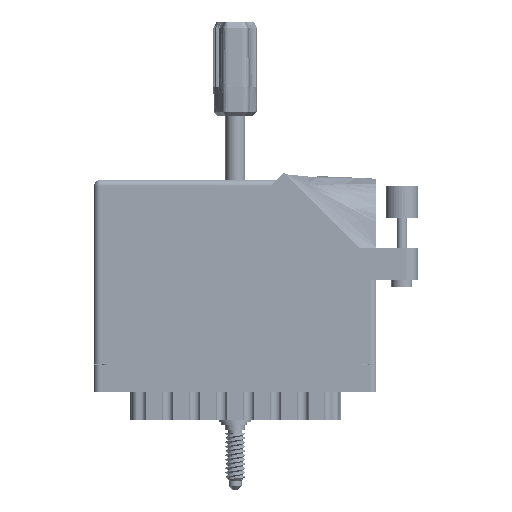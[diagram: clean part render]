
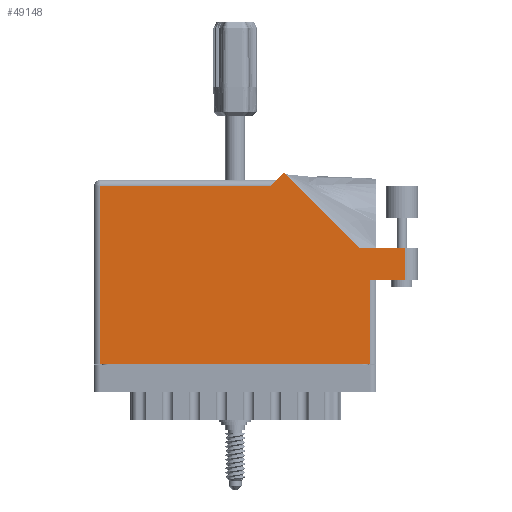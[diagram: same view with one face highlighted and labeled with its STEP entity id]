
A CAD part, front view. The second image highlights one B-rep face of the part: STEP entity #49148.
In plain terms, the highlighted face is planar.
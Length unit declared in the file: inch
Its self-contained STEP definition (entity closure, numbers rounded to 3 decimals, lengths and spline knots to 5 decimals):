
#252 = EDGE_CURVE ( 'NONE', #20971, #59765, #3441, .T. ) ;
#1085 = CARTESIAN_POINT ( 'NONE',  ( 2.55242, 1.122, 0. ) ) ;
#1850 = VECTOR ( 'NONE', #85986, 39.37008 ) ;
#3441 = LINE ( 'NONE', #14086, #82291 ) ;
#5866 = DIRECTION ( 'NONE',  ( 1., 0., 0. ) ) ;
#7881 = VERTEX_POINT ( 'NONE', #88337 ) ;
#8713 = ORIENTED_EDGE ( 'NONE', *, *, #73017, .T. ) ;
#8783 = LINE ( 'NONE', #77100, #63897 ) ;
#11461 = LINE ( 'NONE', #70006, #50453 ) ;
#12929 = VERTEX_POINT ( 'NONE', #83811 ) ;
#14086 = CARTESIAN_POINT ( 'NONE',  ( 2.55242, 1.122, 0. ) ) ;
#16201 = CARTESIAN_POINT ( 'NONE',  ( 1.758, 1.775, 0. ) ) ;
#18513 = CARTESIAN_POINT ( 'NONE',  ( 2.993, 1.122, 0. ) ) ;
#20197 = FACE_OUTER_BOUND ( 'NONE', #36590, .T. ) ;
#20567 = VECTOR ( 'NONE', #42318, 39.37008 ) ;
#20669 = LINE ( 'NONE', #40512, #41167 ) ;
#20687 = VERTEX_POINT ( 'NONE', #79375 ) ;
#20971 = VERTEX_POINT ( 'NONE', #1085 ) ;
#22115 = CARTESIAN_POINT ( 'NONE',  ( 2.656, 0.815, 0. ) ) ;
#22620 = CARTESIAN_POINT ( 'NONE',  ( 0.062, 1.713, 0. ) ) ;
#22723 = CARTESIAN_POINT ( 'NONE',  ( 2.718, 0.815, 0. ) ) ;
#25963 = EDGE_CURVE ( 'NONE', #20687, #50556, #51858, .T. ) ;
#27688 = VECTOR ( 'NONE', #44006, 39.37008 ) ;
#28727 = CARTESIAN_POINT ( 'NONE',  ( 0.062, 0., 0. ) ) ;
#29293 = EDGE_CURVE ( 'NONE', #62999, #12929, #20669, .T. ) ;
#34323 = DIRECTION ( 'NONE',  ( -0.707, 0.707, 0. ) ) ;
#36590 = EDGE_LOOP ( 'NONE', ( #44178, #87037, #39153, #77595, #44686, #8713, #36844, #86407, #63337 ) ) ;
#36844 = ORIENTED_EDGE ( 'NONE', *, *, #80679, .T. ) ;
#39153 = ORIENTED_EDGE ( 'NONE', *, *, #75518, .T. ) ;
#40430 = CARTESIAN_POINT ( 'NONE',  ( 0., 1.713, 0. ) ) ;
#40512 = CARTESIAN_POINT ( 'NONE',  ( 0., 0., 0. ) ) ;
#41167 = VECTOR ( 'NONE', #5866, 39.37008 ) ;
#42318 = DIRECTION ( 'NONE',  ( 1., 0., 0. ) ) ;
#42868 = CARTESIAN_POINT ( 'NONE',  ( 1.82871, 1.84571, 0. ) ) ;
#44006 = DIRECTION ( 'NONE',  ( -1., 0., 0. ) ) ;
#44178 = ORIENTED_EDGE ( 'NONE', *, *, #65555, .T. ) ;
#44686 = ORIENTED_EDGE ( 'NONE', *, *, #80764, .T. ) ;
#49148 = ADVANCED_FACE ( 'NONE', ( #20197 ), #66635, .F. ) ;
#50064 = DIRECTION ( 'NONE',  ( 0., -1., 0. ) ) ;
#50453 = VECTOR ( 'NONE', #50064, 39.37008 ) ;
#50556 = VERTEX_POINT ( 'NONE', #79154 ) ;
#51858 = LINE ( 'NONE', #18513, #77790 ) ;
#53346 = DIRECTION ( 'NONE',  ( -1., 0., 0. ) ) ;
#53641 = CARTESIAN_POINT ( 'NONE',  ( 0., 1.775, 0. ) ) ;
#53952 = DIRECTION ( 'NONE',  ( 0., 0., -1. ) ) ;
#54152 = LINE ( 'NONE', #40430, #82267 ) ;
#59765 = VERTEX_POINT ( 'NONE', #42868 ) ;
#60473 = DIRECTION ( 'NONE',  ( 0., 1., 0. ) ) ;
#61247 = LINE ( 'NONE', #16201, #1850 ) ;
#61403 = AXIS2_PLACEMENT_3D ( 'NONE', #53641, #53952, #53346 ) ;
#62999 = VERTEX_POINT ( 'NONE', #28727 ) ;
#63337 = ORIENTED_EDGE ( 'NONE', *, *, #65035, .T. ) ;
#63897 = VECTOR ( 'NONE', #70153, 39.37008 ) ;
#65035 = EDGE_CURVE ( 'NONE', #12929, #74653, #8783, .T. ) ;
#65555 = EDGE_CURVE ( 'NONE', #74653, #20687, #84390, .T. ) ;
#66635 = PLANE ( 'NONE',  #61403 ) ;
#68007 = VERTEX_POINT ( 'NONE', #22620 ) ;
#70006 = CARTESIAN_POINT ( 'NONE',  ( 0.062, 0., 0. ) ) ;
#70153 = DIRECTION ( 'NONE',  ( 0., 1., 0. ) ) ;
#73017 = EDGE_CURVE ( 'NONE', #7881, #68007, #54152, .T. ) ;
#73193 = LINE ( 'NONE', #86330, #27688 ) ;
#74653 = VERTEX_POINT ( 'NONE', #22115 ) ;
#75518 = EDGE_CURVE ( 'NONE', #50556, #20971, #73193, .T. ) ;
#77100 = CARTESIAN_POINT ( 'NONE',  ( 2.656, 0.815, 0. ) ) ;
#77595 = ORIENTED_EDGE ( 'NONE', *, *, #252, .T. ) ;
#77790 = VECTOR ( 'NONE', #60473, 39.37008 ) ;
#79154 = CARTESIAN_POINT ( 'NONE',  ( 2.993, 1.122, 0. ) ) ;
#79375 = CARTESIAN_POINT ( 'NONE',  ( 2.993, 0.815, 0. ) ) ;
#80679 = EDGE_CURVE ( 'NONE', #68007, #62999, #11461, .T. ) ;
#80764 = EDGE_CURVE ( 'NONE', #59765, #7881, #61247, .T. ) ;
#81890 = DIRECTION ( 'NONE',  ( -1., 0., 0. ) ) ;
#82267 = VECTOR ( 'NONE', #81890, 39.37008 ) ;
#82291 = VECTOR ( 'NONE', #34323, 39.37008 ) ;
#83811 = CARTESIAN_POINT ( 'NONE',  ( 2.656, 0., 0. ) ) ;
#84390 = LINE ( 'NONE', #22723, #20567 ) ;
#85986 = DIRECTION ( 'NONE',  ( -0.707, -0.707, 0. ) ) ;
#86330 = CARTESIAN_POINT ( 'NONE',  ( 3.118, 1.122, 0. ) ) ;
#86407 = ORIENTED_EDGE ( 'NONE', *, *, #29293, .T. ) ;
#87037 = ORIENTED_EDGE ( 'NONE', *, *, #25963, .T. ) ;
#88337 = CARTESIAN_POINT ( 'NONE',  ( 1.696, 1.713, 0. ) ) ;
